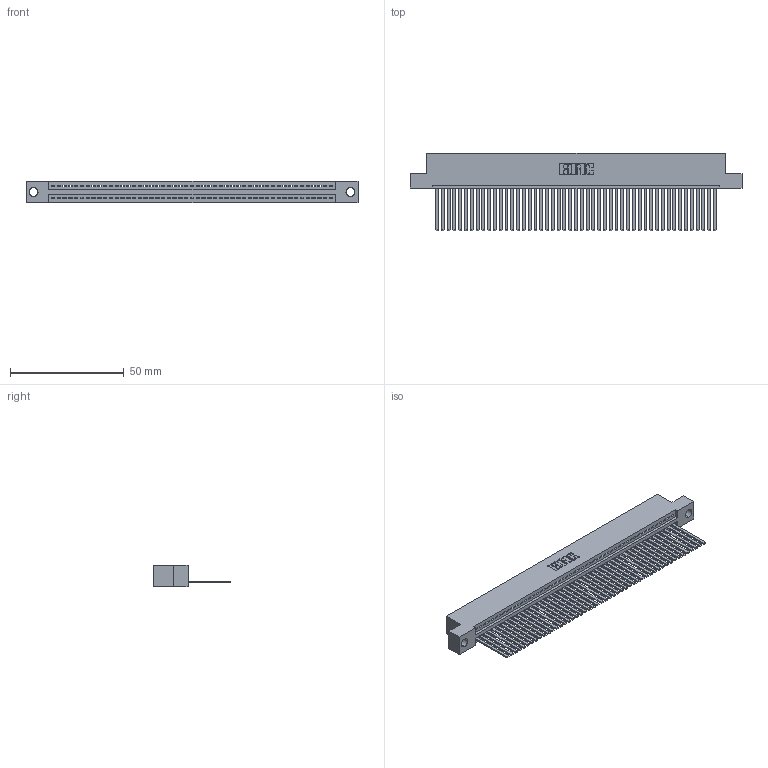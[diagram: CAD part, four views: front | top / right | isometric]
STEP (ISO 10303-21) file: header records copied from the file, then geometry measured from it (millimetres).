
FILE_DESCRIPTION (( 'STEP AP203' ), '1' );
FILE_NAME ('345-049-544-104.STEP', '2019-10-09T09:31:15', ( '' ), ( '' ), 'SwSTEP 2.0', 'SolidWorks 2016', '' );
FILE_SCHEMA (( 'CONFIG_CONTROL_DESIGN' ));
Length unit declared in the file: inch
Products named in the file (3): 345 Part_Flush Mounting Lugs - 0.156 Dia-TH; 345-292-001_345-293-144; 345-049-544-104
Assembly tree (50 placements, depth 2):
  345-049-544-104
    345 Part_Flush Mounting Lugs - 0.156 Dia-TH
    345-292-001_345-293-144  x49
Bounding box: 145.67 x 33.96 x 9.4 mm (x, y, z)
Volume: 14372.8 mm3; surface area: 20707.6 mm2
Topology: 50 solids, 50 shells, 2674 faces, 8083 edges, 5322 vertices
Faces by surface type: plane 1844, cylinder 830
Entity records: 35755 total; most frequent: CARTESIAN_POINT 6199, ORIENTED_EDGE 6182, DIRECTION 5401, EDGE_CURVE 3091, LINE 2767, VECTOR 2767, VERTEX_POINT 2058, AXIS2_PLACEMENT_3D 1317
